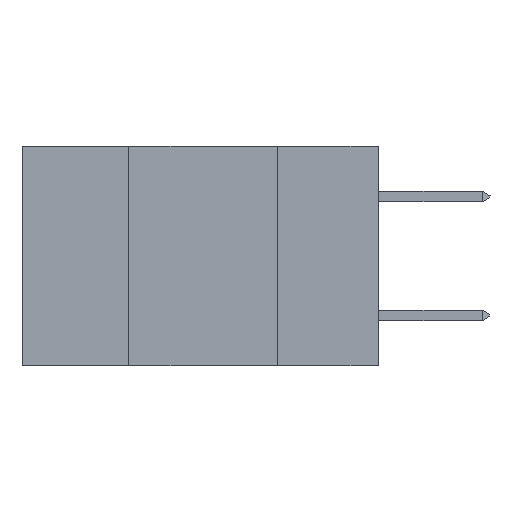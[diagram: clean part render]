
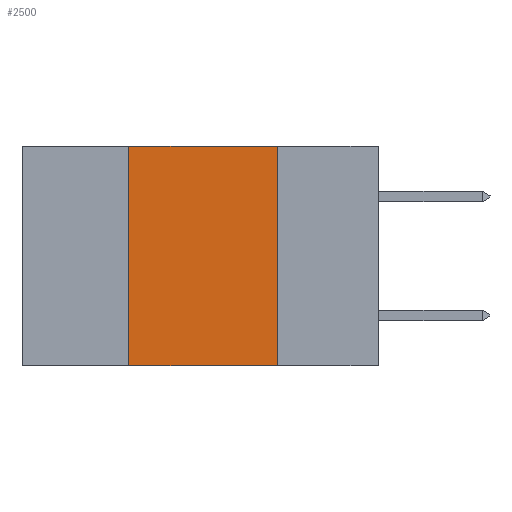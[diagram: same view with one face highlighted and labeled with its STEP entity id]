
A CAD part, left-side view. The second image highlights one B-rep face of the part: STEP entity #2500.
In plain terms, the highlighted planar face has unit normal (-1, 0, 0).
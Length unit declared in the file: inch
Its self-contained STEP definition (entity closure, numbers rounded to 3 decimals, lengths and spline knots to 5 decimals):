
#1451 = CARTESIAN_POINT ( 'NONE',  ( 0., 0.17, 0. ) ) ;
#2197 = ORIENTED_EDGE ( 'NONE', *, *, #16994, .F. ) ;
#2500 = ADVANCED_FACE ( 'NONE', ( #26380 ), #22397, .F. ) ;
#3385 = VECTOR ( 'NONE', #11070, 39.37008 ) ;
#3883 = EDGE_CURVE ( 'NONE', #9062, #25771, #16271, .T. ) ;
#5789 = DIRECTION ( 'NONE',  ( 0., -1., 0. ) ) ;
#6430 = CARTESIAN_POINT ( 'NONE',  ( 0., 0.42, 0. ) ) ;
#6832 = DIRECTION ( 'NONE',  ( 0., 0., 1. ) ) ;
#7304 = AXIS2_PLACEMENT_3D ( 'NONE', #14100, #7837, #10268 ) ;
#7605 = VECTOR ( 'NONE', #6832, 39.37008 ) ;
#7837 = DIRECTION ( 'NONE',  ( 1., 0., 0. ) ) ;
#8886 = LINE ( 'NONE', #21415, #3385 ) ;
#9062 = VERTEX_POINT ( 'NONE', #1451 ) ;
#9315 = EDGE_CURVE ( 'NONE', #24388, #9062, #8886, .T. ) ;
#9918 = CARTESIAN_POINT ( 'NONE',  ( 0., 0.42, -0.37 ) ) ;
#10268 = DIRECTION ( 'NONE',  ( 0., 0., -1. ) ) ;
#10785 = CARTESIAN_POINT ( 'NONE',  ( 0., 0.42, -0.37 ) ) ;
#11070 = DIRECTION ( 'NONE',  ( 0., -1., 0. ) ) ;
#12317 = CARTESIAN_POINT ( 'NONE',  ( 0., 0.17, -0.37 ) ) ;
#12883 = ORIENTED_EDGE ( 'NONE', *, *, #3883, .F. ) ;
#13694 = CARTESIAN_POINT ( 'NONE',  ( 0., 0.17, -0.37 ) ) ;
#13892 = EDGE_LOOP ( 'NONE', ( #12883, #23840, #2197, #19230 ) ) ;
#14100 = CARTESIAN_POINT ( 'NONE',  ( 0., 0.6, 0. ) ) ;
#16144 = LINE ( 'NONE', #24458, #21934 ) ;
#16271 = LINE ( 'NONE', #12317, #22510 ) ;
#16544 = DIRECTION ( 'NONE',  ( 0., 0., -1. ) ) ;
#16994 = EDGE_CURVE ( 'NONE', #26652, #24388, #21534, .T. ) ;
#19230 = ORIENTED_EDGE ( 'NONE', *, *, #23790, .T. ) ;
#21415 = CARTESIAN_POINT ( 'NONE',  ( 0., 0.6, 0. ) ) ;
#21534 = LINE ( 'NONE', #10785, #7605 ) ;
#21934 = VECTOR ( 'NONE', #5789, 39.37008 ) ;
#22397 = PLANE ( 'NONE',  #7304 ) ;
#22510 = VECTOR ( 'NONE', #16544, 39.37008 ) ;
#23790 = EDGE_CURVE ( 'NONE', #26652, #25771, #16144, .T. ) ;
#23840 = ORIENTED_EDGE ( 'NONE', *, *, #9315, .F. ) ;
#24388 = VERTEX_POINT ( 'NONE', #6430 ) ;
#24458 = CARTESIAN_POINT ( 'NONE',  ( 0., 0.6, -0.37 ) ) ;
#25771 = VERTEX_POINT ( 'NONE', #13694 ) ;
#26380 = FACE_OUTER_BOUND ( 'NONE', #13892, .T. ) ;
#26652 = VERTEX_POINT ( 'NONE', #9918 ) ;
